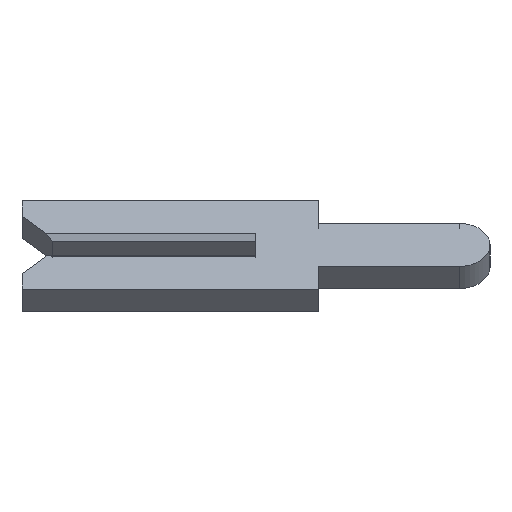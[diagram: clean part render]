
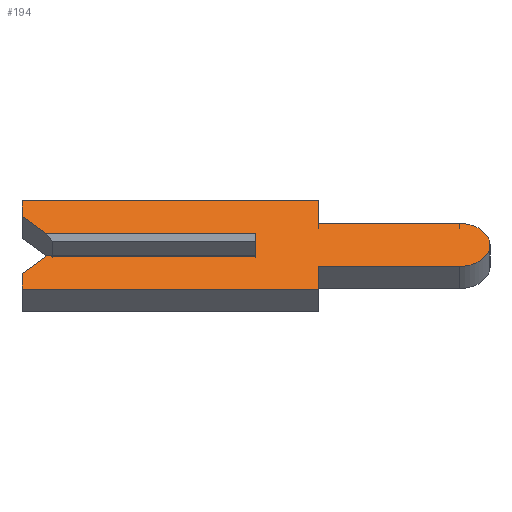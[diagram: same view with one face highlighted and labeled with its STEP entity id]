
A CAD part, left-side view. The second image highlights one B-rep face of the part: STEP entity #194.
In plain terms, the highlighted face is planar.
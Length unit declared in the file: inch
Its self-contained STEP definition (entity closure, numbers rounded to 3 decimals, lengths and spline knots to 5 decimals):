
#2 = CARTESIAN_POINT ( 'NONE',  ( -0.01, -0.1305, 0. ) ) ;
#22 = VECTOR ( 'NONE', #1310, 39.37008 ) ;
#34 = VERTEX_POINT ( 'NONE', #418 ) ;
#35 = CIRCLE ( 'NONE', #476, 0.0195 ) ;
#39 = CARTESIAN_POINT ( 'NONE',  ( -0.01, -0.1305, -0.01 ) ) ;
#51 = CARTESIAN_POINT ( 'NONE',  ( -0.01, -0.04, 0.04 ) ) ;
#64 = EDGE_CURVE ( 'NONE', #282, #193, #35, .T. ) ;
#65 = FACE_OUTER_BOUND ( 'NONE', #281, .T. ) ;
#81 = CARTESIAN_POINT ( 'NONE',  ( -0.01, 0.15, 0.026 ) ) ;
#84 = CARTESIAN_POINT ( 'NONE',  ( -0.01, 0.15, 0.01 ) ) ;
#102 = CARTESIAN_POINT ( 'NONE',  ( -0.01, -0.04, -0.04 ) ) ;
#114 = VERTEX_POINT ( 'NONE', #102 ) ;
#115 = DIRECTION ( 'NONE',  ( 0., 0., 1. ) ) ;
#116 = LINE ( 'NONE', #1295, #509 ) ;
#131 = DIRECTION ( 'NONE',  ( 0., 1., 0. ) ) ;
#132 = ORIENTED_EDGE ( 'NONE', *, *, #934, .F. ) ;
#177 = ORIENTED_EDGE ( 'NONE', *, *, #957, .T. ) ;
#192 = CARTESIAN_POINT ( 'NONE',  ( -0.01, 0.1305, 0.0065 ) ) ;
#193 = VERTEX_POINT ( 'NONE', #542 ) ;
#194 = ADVANCED_FACE ( 'NONE', ( #65 ), #212, .F. ) ;
#210 = EDGE_CURVE ( 'NONE', #1253, #529, #643, .T. ) ;
#212 = PLANE ( 'NONE',  #1173 ) ;
#222 = DIRECTION ( 'NONE',  ( 0., 0., -1. ) ) ;
#230 = LINE ( 'NONE', #84, #352 ) ;
#235 = DIRECTION ( 'NONE',  ( 0., -0.707, 0.707 ) ) ;
#248 = VERTEX_POINT ( 'NONE', #310 ) ;
#257 = EDGE_CURVE ( 'NONE', #675, #114, #116, .T. ) ;
#272 = CARTESIAN_POINT ( 'NONE',  ( -0.01, -0.04, -0.0195 ) ) ;
#274 = VECTOR ( 'NONE', #235, 39.37008 ) ;
#279 = VECTOR ( 'NONE', #1360, 39.37008 ) ;
#281 = EDGE_LOOP ( 'NONE', ( #177, #1370, #386, #688, #1127, #1089, #1288, #719, #1103, #1270, #1125, #601, #1209, #132 ) ) ;
#282 = VERTEX_POINT ( 'NONE', #986 ) ;
#296 = LINE ( 'NONE', #192, #279 ) ;
#299 = VECTOR ( 'NONE', #506, 39.37008 ) ;
#310 = CARTESIAN_POINT ( 'NONE',  ( -0.01, 0.15, 0.04 ) ) ;
#321 = VERTEX_POINT ( 'NONE', #458 ) ;
#322 = CARTESIAN_POINT ( 'NONE',  ( -0.01, -0.04, 0.0195 ) ) ;
#352 = VECTOR ( 'NONE', #520, 39.37008 ) ;
#353 = EDGE_CURVE ( 'NONE', #248, #722, #602, .T. ) ;
#357 = CARTESIAN_POINT ( 'NONE',  ( -0.01, -0.04, -0.0195 ) ) ;
#373 = EDGE_CURVE ( 'NONE', #193, #675, #757, .T. ) ;
#386 = ORIENTED_EDGE ( 'NONE', *, *, #550, .F. ) ;
#390 = DIRECTION ( 'NONE',  ( 0., 1., 0. ) ) ;
#394 = EDGE_CURVE ( 'NONE', #34, #1253, #474, .T. ) ;
#399 = CARTESIAN_POINT ( 'NONE',  ( -0.01, -0.04, 0.0195 ) ) ;
#403 = CARTESIAN_POINT ( 'NONE',  ( -0.01, 0., 0.0065 ) ) ;
#418 = CARTESIAN_POINT ( 'NONE',  ( -0.01, 0.15, -0.04 ) ) ;
#442 = EDGE_CURVE ( 'NONE', #997, #248, #510, .T. ) ;
#450 = CARTESIAN_POINT ( 'NONE',  ( -0.01, 0.15, -0.026 ) ) ;
#458 = CARTESIAN_POINT ( 'NONE',  ( -0.01, 0., -0.01 ) ) ;
#474 = LINE ( 'NONE', #450, #1068 ) ;
#476 = AXIS2_PLACEMENT_3D ( 'NONE', #2, #744, #222 ) ;
#506 = DIRECTION ( 'NONE',  ( 0., -1., 0. ) ) ;
#509 = VECTOR ( 'NONE', #676, 39.37008 ) ;
#510 = LINE ( 'NONE', #581, #533 ) ;
#520 = DIRECTION ( 'NONE',  ( 0., -1., 0. ) ) ;
#522 = DIRECTION ( 'NONE',  ( 0., 0., -1. ) ) ;
#523 = VECTOR ( 'NONE', #522, 39.37008 ) ;
#529 = VERTEX_POINT ( 'NONE', #1014 ) ;
#533 = VECTOR ( 'NONE', #115, 39.37008 ) ;
#534 = VECTOR ( 'NONE', #933, 39.37008 ) ;
#542 = CARTESIAN_POINT ( 'NONE',  ( -0.01, -0.1305, -0.0195 ) ) ;
#543 = CARTESIAN_POINT ( 'NONE',  ( -0.01, 0., 0.01 ) ) ;
#546 = DIRECTION ( 'NONE',  ( 1., 0., 0. ) ) ;
#550 = EDGE_CURVE ( 'NONE', #529, #321, #778, .T. ) ;
#581 = CARTESIAN_POINT ( 'NONE',  ( -0.01, 0.15, 0.026 ) ) ;
#601 = ORIENTED_EDGE ( 'NONE', *, *, #353, .F. ) ;
#602 = LINE ( 'NONE', #1082, #22 ) ;
#620 = VECTOR ( 'NONE', #390, 39.37008 ) ;
#643 = LINE ( 'NONE', #772, #274 ) ;
#675 = VERTEX_POINT ( 'NONE', #272 ) ;
#676 = DIRECTION ( 'NONE',  ( 0., 0., -1. ) ) ;
#688 = ORIENTED_EDGE ( 'NONE', *, *, #210, .F. ) ;
#714 = CARTESIAN_POINT ( 'NONE',  ( -0.01, 0.15, -0.04 ) ) ;
#717 = VERTEX_POINT ( 'NONE', #1008 ) ;
#719 = ORIENTED_EDGE ( 'NONE', *, *, #373, .F. ) ;
#722 = VERTEX_POINT ( 'NONE', #51 ) ;
#744 = DIRECTION ( 'NONE',  ( 1., 0., 0. ) ) ;
#757 = LINE ( 'NONE', #357, #999 ) ;
#772 = CARTESIAN_POINT ( 'NONE',  ( -0.01, 0.1305, -0.0065 ) ) ;
#778 = LINE ( 'NONE', #39, #1198 ) ;
#861 = EDGE_CURVE ( 'NONE', #114, #34, #1187, .T. ) ;
#862 = CARTESIAN_POINT ( 'NONE',  ( -0.01, 0.15, -0.026 ) ) ;
#878 = DIRECTION ( 'NONE',  ( 0., 0., 1. ) ) ;
#887 = EDGE_CURVE ( 'NONE', #1190, #282, #1155, .T. ) ;
#933 = DIRECTION ( 'NONE',  ( 0., 0., 1. ) ) ;
#934 = EDGE_CURVE ( 'NONE', #717, #997, #296, .T. ) ;
#943 = EDGE_CURVE ( 'NONE', #722, #1190, #1028, .T. ) ;
#947 = LINE ( 'NONE', #403, #534 ) ;
#949 = CARTESIAN_POINT ( 'NONE',  ( -0.01, -0.1305, 0. ) ) ;
#954 = DIRECTION ( 'NONE',  ( 0., 0., -1. ) ) ;
#957 = EDGE_CURVE ( 'NONE', #717, #1317, #230, .T. ) ;
#986 = CARTESIAN_POINT ( 'NONE',  ( -0.01, -0.1305, 0.0195 ) ) ;
#997 = VERTEX_POINT ( 'NONE', #81 ) ;
#999 = VECTOR ( 'NONE', #131, 39.37008 ) ;
#1008 = CARTESIAN_POINT ( 'NONE',  ( -0.01, 0.134, 0.01 ) ) ;
#1014 = CARTESIAN_POINT ( 'NONE',  ( -0.01, 0.134, -0.01 ) ) ;
#1028 = LINE ( 'NONE', #1274, #523 ) ;
#1068 = VECTOR ( 'NONE', #878, 39.37008 ) ;
#1082 = CARTESIAN_POINT ( 'NONE',  ( -0.01, 0.15, 0.04 ) ) ;
#1089 = ORIENTED_EDGE ( 'NONE', *, *, #861, .F. ) ;
#1103 = ORIENTED_EDGE ( 'NONE', *, *, #64, .F. ) ;
#1125 = ORIENTED_EDGE ( 'NONE', *, *, #943, .F. ) ;
#1127 = ORIENTED_EDGE ( 'NONE', *, *, #394, .F. ) ;
#1145 = EDGE_CURVE ( 'NONE', #321, #1317, #947, .T. ) ;
#1155 = LINE ( 'NONE', #399, #299 ) ;
#1173 = AXIS2_PLACEMENT_3D ( 'NONE', #949, #546, #954 ) ;
#1187 = LINE ( 'NONE', #714, #620 ) ;
#1190 = VERTEX_POINT ( 'NONE', #322 ) ;
#1198 = VECTOR ( 'NONE', #1216, 39.37008 ) ;
#1209 = ORIENTED_EDGE ( 'NONE', *, *, #442, .F. ) ;
#1216 = DIRECTION ( 'NONE',  ( 0., -1., 0. ) ) ;
#1253 = VERTEX_POINT ( 'NONE', #862 ) ;
#1270 = ORIENTED_EDGE ( 'NONE', *, *, #887, .F. ) ;
#1274 = CARTESIAN_POINT ( 'NONE',  ( -0.01, -0.04, 0.04 ) ) ;
#1288 = ORIENTED_EDGE ( 'NONE', *, *, #257, .F. ) ;
#1295 = CARTESIAN_POINT ( 'NONE',  ( -0.01, -0.04, -0.04 ) ) ;
#1310 = DIRECTION ( 'NONE',  ( 0., -1., 0. ) ) ;
#1317 = VERTEX_POINT ( 'NONE', #543 ) ;
#1360 = DIRECTION ( 'NONE',  ( 0., 0.707, 0.707 ) ) ;
#1370 = ORIENTED_EDGE ( 'NONE', *, *, #1145, .F. ) ;
